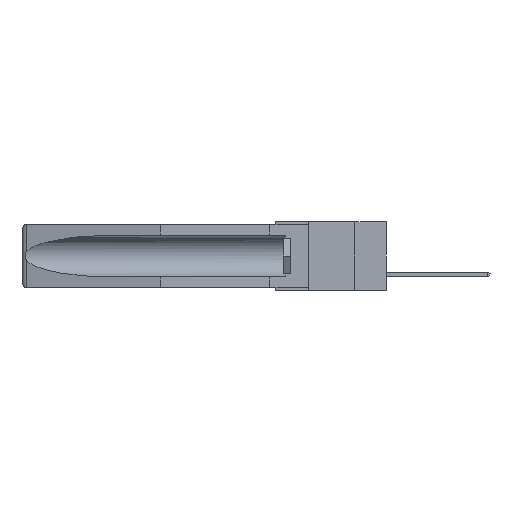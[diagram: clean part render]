
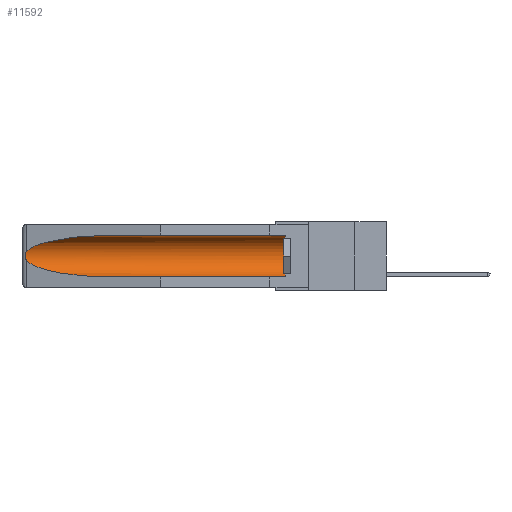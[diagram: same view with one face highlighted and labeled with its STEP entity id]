
A CAD part, left-side view. The second image highlights one B-rep face of the part: STEP entity #11592.
In plain terms, the highlighted cylindrical face has radius 2.857 mm (diameter 5.715 mm), a partial arc.
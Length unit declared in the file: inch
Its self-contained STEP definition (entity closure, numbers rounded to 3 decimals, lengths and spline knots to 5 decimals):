
#23 = B_SPLINE_CURVE_WITH_KNOTS ( 'NONE', 3,
 ( #17774, #4960, #10717, #17840, #17965, #16549, #3550, #16352, #16480, #7883 ),
 .UNSPECIFIED., .F., .F.,
 ( 4, 2, 2, 2, 4 ),
 ( 0., 0.00029, 0.00058, 0.00087, 0.00117 ),
 .UNSPECIFIED. ) ;
#634 = LINE ( 'NONE', #13629, #7300 ) ;
#924 = AXIS2_PLACEMENT_3D ( 'NONE', #9718, #1203, #16927 ) ;
#1203 = DIRECTION ( 'NONE',  ( 0., 1., 0. ) ) ;
#3110 = ORIENTED_EDGE ( 'NONE', *, *, #5907, .T. ) ;
#3250 = CARTESIAN_POINT ( 'NONE',  ( 0.25451, 1.48313, -0.24835 ) ) ;
#3550 = CARTESIAN_POINT ( 'NONE',  ( 0.2673, 1.53269, -0.17917 ) ) ;
#3557 = VERTEX_POINT ( 'NONE', #9167 ) ;
#4153 = CARTESIAN_POINT ( 'NONE',  ( 0.155, -0.30754, -0.059 ) ) ;
#4524 = CARTESIAN_POINT ( 'NONE',  ( 0.26537, 1.52718, -0.14972 ) ) ;
#4569 = EDGE_CURVE ( 'NONE', #6914, #9357, #634, .T. ) ;
#4657 = DIRECTION ( 'NONE',  ( 0., -1., 0. ) ) ;
#4960 = CARTESIAN_POINT ( 'NONE',  ( 0.26597, 1.52961, -0.15275 ) ) ;
#5730 = AXIS2_PLACEMENT_3D ( 'NONE', #16098, #4657, #17471 ) ;
#5797 = EDGE_CURVE ( 'NONE', #6914, #17301, #12215, .T. ) ;
#5907 = EDGE_CURVE ( 'NONE', #14173, #3557, #23, .T. ) ;
#5927 = CARTESIAN_POINT ( 'NONE',  ( 0.26537, 1.52718, -0.19328 ) ) ;
#6630 = DIRECTION ( 'NONE',  ( 0., 1., 0. ) ) ;
#6829 = CARTESIAN_POINT ( 'NONE',  ( 0.155, 1.07973, -0.059 ) ) ;
#6914 = VERTEX_POINT ( 'NONE', #9013 ) ;
#6952 = EDGE_CURVE ( 'NONE', #17301, #8033, #11510, .T. ) ;
#7300 = VECTOR ( 'NONE', #7683, 39.37008 ) ;
#7354 = CARTESIAN_POINT ( 'NONE',  ( 0.21114, 1.30732, -0.284 ) ) ;
#7683 = DIRECTION ( 'NONE',  ( 0., 1., 0. ) ) ;
#7883 = CARTESIAN_POINT ( 'NONE',  ( 0.26537, 1.52718, -0.19328 ) ) ;
#8033 = VERTEX_POINT ( 'NONE', #6829 ) ;
#8786 = ORIENTED_EDGE ( 'NONE', *, *, #12950, .T. ) ;
#8884 = CARTESIAN_POINT ( 'NONE',  ( 0.25451, 1.48313, -0.09465 ) ) ;
#8936 = CARTESIAN_POINT ( 'NONE',  ( 0.155, 0.126, -0.059 ) ) ;
#9013 = CARTESIAN_POINT ( 'NONE',  ( 0.155, 0.126, -0.284 ) ) ;
#9081 = FACE_OUTER_BOUND ( 'NONE', #11544, .T. ) ;
#9167 = CARTESIAN_POINT ( 'NONE',  ( 0.26537, 1.52718, -0.19328 ) ) ;
#9357 = VERTEX_POINT ( 'NONE', #12866 ) ;
#9378 =( BOUNDED_CURVE ( )  B_SPLINE_CURVE ( 3, ( #15959, #11771, #8884, #4524 ),
 .UNSPECIFIED., .F., .F. ) 
 B_SPLINE_CURVE_WITH_KNOTS ( ( 4, 4 ),
 ( 4.71239, 6.08839 ),
 .UNSPECIFIED. ) 
 CURVE ( )  GEOMETRIC_REPRESENTATION_ITEM ( )  RATIONAL_B_SPLINE_CURVE ( ( 1., 0.848, 0.848, 1. ) ) 
 REPRESENTATION_ITEM ( '' )  );
#9508 = EDGE_CURVE ( 'NONE', #3557, #9357, #14421, .T. ) ;
#9718 = CARTESIAN_POINT ( 'NONE',  ( 0.155, -0.30754, -0.1715 ) ) ;
#10346 = ORIENTED_EDGE ( 'NONE', *, *, #6952, .T. ) ;
#10717 = CARTESIAN_POINT ( 'NONE',  ( 0.26654, 1.53092, -0.15636 ) ) ;
#11510 = LINE ( 'NONE', #4153, #12187 ) ;
#11544 = EDGE_LOOP ( 'NONE', ( #8786, #3110, #18176, #11721, #11747, #10346 ) ) ;
#11592 = ADVANCED_FACE ( 'NONE', ( #9081 ), #16261, .F. ) ;
#11721 = ORIENTED_EDGE ( 'NONE', *, *, #4569, .F. ) ;
#11747 = ORIENTED_EDGE ( 'NONE', *, *, #5797, .T. ) ;
#11771 = CARTESIAN_POINT ( 'NONE',  ( 0.21114, 1.30732, -0.059 ) ) ;
#12187 = VECTOR ( 'NONE', #6630, 39.37008 ) ;
#12215 = CIRCLE ( 'NONE', #5730, 0.1125 ) ;
#12866 = CARTESIAN_POINT ( 'NONE',  ( 0.155, 1.07973, -0.284 ) ) ;
#12950 = EDGE_CURVE ( 'NONE', #8033, #14173, #9378, .T. ) ;
#13629 = CARTESIAN_POINT ( 'NONE',  ( 0.155, -0.30754, -0.284 ) ) ;
#14173 = VERTEX_POINT ( 'NONE', #18157 ) ;
#14421 =( BOUNDED_CURVE ( )  B_SPLINE_CURVE ( 3, ( #5927, #3250, #7354, #16116 ),
 .UNSPECIFIED., .F., .F. ) 
 B_SPLINE_CURVE_WITH_KNOTS ( ( 4, 4 ),
 ( 0.1948, 1.5708 ),
 .UNSPECIFIED. ) 
 CURVE ( )  GEOMETRIC_REPRESENTATION_ITEM ( )  RATIONAL_B_SPLINE_CURVE ( ( 1., 0.848, 0.848, 1. ) ) 
 REPRESENTATION_ITEM ( '' )  );
#15959 = CARTESIAN_POINT ( 'NONE',  ( 0.155, 1.07973, -0.059 ) ) ;
#16098 = CARTESIAN_POINT ( 'NONE',  ( 0.155, 0.126, -0.1715 ) ) ;
#16116 = CARTESIAN_POINT ( 'NONE',  ( 0.155, 1.07973, -0.284 ) ) ;
#16261 = CYLINDRICAL_SURFACE ( 'NONE', #924, 0.1125 ) ;
#16352 = CARTESIAN_POINT ( 'NONE',  ( 0.26655, 1.53094, -0.18657 ) ) ;
#16480 = CARTESIAN_POINT ( 'NONE',  ( 0.26597, 1.5296, -0.19026 ) ) ;
#16549 = CARTESIAN_POINT ( 'NONE',  ( 0.2675, 1.53308, -0.17534 ) ) ;
#16927 = DIRECTION ( 'NONE',  ( 0., 0., 1. ) ) ;
#17301 = VERTEX_POINT ( 'NONE', #8936 ) ;
#17471 = DIRECTION ( 'NONE',  ( 0., 0., 1. ) ) ;
#17774 = CARTESIAN_POINT ( 'NONE',  ( 0.26537, 1.52718, -0.14972 ) ) ;
#17840 = CARTESIAN_POINT ( 'NONE',  ( 0.2673, 1.5327, -0.16383 ) ) ;
#17965 = CARTESIAN_POINT ( 'NONE',  ( 0.2675, 1.53308, -0.16763 ) ) ;
#18157 = CARTESIAN_POINT ( 'NONE',  ( 0.26537, 1.52718, -0.14972 ) ) ;
#18176 = ORIENTED_EDGE ( 'NONE', *, *, #9508, .T. ) ;
